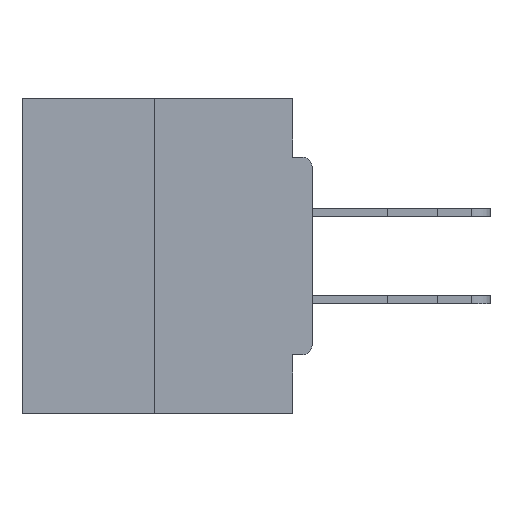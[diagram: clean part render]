
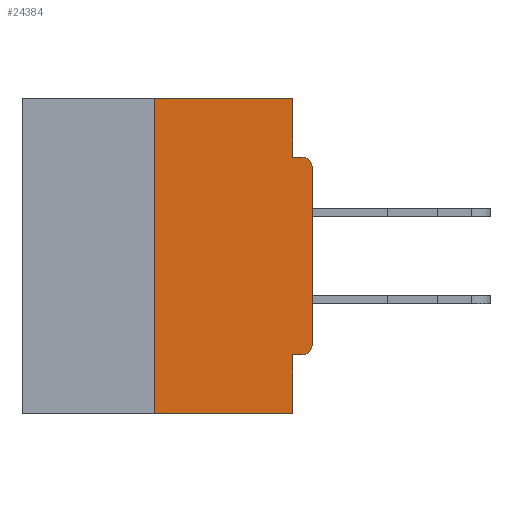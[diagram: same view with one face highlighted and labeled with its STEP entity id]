
A CAD part, left-side view. The second image highlights one B-rep face of the part: STEP entity #24384.
In plain terms, the highlighted planar face has unit normal (-1, 0, 0).
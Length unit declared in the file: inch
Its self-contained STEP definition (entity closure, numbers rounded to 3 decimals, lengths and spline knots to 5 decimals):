
#837 = DIRECTION ( 'NONE',  ( 0., 0., -1. ) ) ;
#1456 = LINE ( 'NONE', #22021, #6409 ) ;
#1911 = AXIS2_PLACEMENT_3D ( 'NONE', #15121, #15241, #32262 ) ;
#2408 = DIRECTION ( 'NONE',  ( 0., 0., -1. ) ) ;
#2849 = CARTESIAN_POINT ( 'NONE',  ( 0., 0.031, -0.4065 ) ) ;
#3542 = VECTOR ( 'NONE', #2408, 39.37008 ) ;
#3547 = VERTEX_POINT ( 'NONE', #22364 ) ;
#3574 = DIRECTION ( 'NONE',  ( -1., 0., 0. ) ) ;
#3771 = DIRECTION ( 'NONE',  ( 0., 1., 0. ) ) ;
#4537 = ORIENTED_EDGE ( 'NONE', *, *, #19357, .F. ) ;
#5970 = VERTEX_POINT ( 'NONE', #33038 ) ;
#6409 = VECTOR ( 'NONE', #3771, 39.37008 ) ;
#6450 = VECTOR ( 'NONE', #30759, 39.37008 ) ;
#7150 = DIRECTION ( 'NONE',  ( 0., 0., 1. ) ) ;
#7589 = LINE ( 'NONE', #16552, #3542 ) ;
#7725 = CARTESIAN_POINT ( 'NONE',  ( 0., 0.46, -0.5 ) ) ;
#9317 = DIRECTION ( 'NONE',  ( 0., -1., 0. ) ) ;
#9346 = EDGE_CURVE ( 'NONE', #17572, #32193, #27491, .T. ) ;
#9923 = ORIENTED_EDGE ( 'NONE', *, *, #14811, .T. ) ;
#10273 = ORIENTED_EDGE ( 'NONE', *, *, #27734, .F. ) ;
#11544 = LINE ( 'NONE', #16419, #13365 ) ;
#11644 = DIRECTION ( 'NONE',  ( 0., -1., 0. ) ) ;
#11818 = LINE ( 'NONE', #21107, #30817 ) ;
#12034 = CARTESIAN_POINT ( 'NONE',  ( 0., 0., -0.3915 ) ) ;
#12167 = AXIS2_PLACEMENT_3D ( 'NONE', #26490, #3574, #837 ) ;
#12529 = DIRECTION ( 'NONE',  ( 0., 0., -1. ) ) ;
#13314 = EDGE_CURVE ( 'NONE', #35030, #5970, #11818, .T. ) ;
#13365 = VECTOR ( 'NONE', #30950, 39.37008 ) ;
#14696 = CARTESIAN_POINT ( 'NONE',  ( 0., 0.015, -0.4065 ) ) ;
#14811 = EDGE_CURVE ( 'NONE', #3547, #5970, #28433, .T. ) ;
#15121 = CARTESIAN_POINT ( 'NONE',  ( 0., 0.015, -0.3915 ) ) ;
#15241 = DIRECTION ( 'NONE',  ( -1., 0., 0. ) ) ;
#15421 = PLANE ( 'NONE',  #22726 ) ;
#16419 = CARTESIAN_POINT ( 'NONE',  ( 0., 0., 0. ) ) ;
#16548 = LINE ( 'NONE', #17117, #25144 ) ;
#16552 = CARTESIAN_POINT ( 'NONE',  ( 0., 0.031, 0. ) ) ;
#16988 = DIRECTION ( 'NONE',  ( 0., 0., -1. ) ) ;
#17117 = CARTESIAN_POINT ( 'NONE',  ( 0., 0.031, -0.5 ) ) ;
#17572 = VERTEX_POINT ( 'NONE', #14696 ) ;
#19357 = EDGE_CURVE ( 'NONE', #35342, #22107, #31968, .T. ) ;
#19617 = VECTOR ( 'NONE', #11644, 39.37008 ) ;
#19717 = EDGE_CURVE ( 'NONE', #37078, #26133, #16548, .T. ) ;
#21019 = LINE ( 'NONE', #26024, #19617 ) ;
#21107 = CARTESIAN_POINT ( 'NONE',  ( 0., 0., -0.0935 ) ) ;
#21246 = ORIENTED_EDGE ( 'NONE', *, *, #9346, .T. ) ;
#21857 = ORIENTED_EDGE ( 'NONE', *, *, #22787, .F. ) ;
#22021 = CARTESIAN_POINT ( 'NONE',  ( 0., 0., -0.4065 ) ) ;
#22107 = VERTEX_POINT ( 'NONE', #24955 ) ;
#22237 = CARTESIAN_POINT ( 'NONE',  ( 0., 0.031, -0.5 ) ) ;
#22364 = CARTESIAN_POINT ( 'NONE',  ( 0., 0., -0.1085 ) ) ;
#22726 = AXIS2_PLACEMENT_3D ( 'NONE', #24101, #32914, #12529 ) ;
#22787 = EDGE_CURVE ( 'NONE', #17572, #37078, #1456, .T. ) ;
#23242 = ORIENTED_EDGE ( 'NONE', *, *, #13314, .F. ) ;
#24101 = CARTESIAN_POINT ( 'NONE',  ( 0., 0.46, 0. ) ) ;
#24384 = ADVANCED_FACE ( 'NONE', ( #34598 ), #15421, .F. ) ;
#24397 = CARTESIAN_POINT ( 'NONE',  ( 0., 0.031, 0. ) ) ;
#24955 = CARTESIAN_POINT ( 'NONE',  ( 0., 0.25, 0. ) ) ;
#25144 = VECTOR ( 'NONE', #16988, 39.37008 ) ;
#25373 = CARTESIAN_POINT ( 'NONE',  ( 0., 0.031, -0.0935 ) ) ;
#26024 = CARTESIAN_POINT ( 'NONE',  ( 0., 0.46, 0. ) ) ;
#26133 = VERTEX_POINT ( 'NONE', #22237 ) ;
#26490 = CARTESIAN_POINT ( 'NONE',  ( 0., 0.015, -0.1085 ) ) ;
#26702 = LINE ( 'NONE', #7725, #6450 ) ;
#27491 = CIRCLE ( 'NONE', #1911, 0.015 ) ;
#27734 = EDGE_CURVE ( 'NONE', #34871, #35030, #7589, .T. ) ;
#28433 = CIRCLE ( 'NONE', #12167, 0.015 ) ;
#29302 = EDGE_CURVE ( 'NONE', #22107, #34871, #21019, .T. ) ;
#30649 = CARTESIAN_POINT ( 'NONE',  ( 0., 0.25, -0.5 ) ) ;
#30711 = ORIENTED_EDGE ( 'NONE', *, *, #29302, .F. ) ;
#30759 = DIRECTION ( 'NONE',  ( 0., -1., 0. ) ) ;
#30817 = VECTOR ( 'NONE', #9317, 39.37008 ) ;
#30950 = DIRECTION ( 'NONE',  ( 0., 0., 1. ) ) ;
#31752 = EDGE_CURVE ( 'NONE', #35342, #26133, #26702, .T. ) ;
#31968 = LINE ( 'NONE', #36042, #35516 ) ;
#32193 = VERTEX_POINT ( 'NONE', #12034 ) ;
#32262 = DIRECTION ( 'NONE',  ( 0., 0., -1. ) ) ;
#32849 = ORIENTED_EDGE ( 'NONE', *, *, #31752, .T. ) ;
#32914 = DIRECTION ( 'NONE',  ( 1., 0., 0. ) ) ;
#33038 = CARTESIAN_POINT ( 'NONE',  ( 0., 0.015, -0.0935 ) ) ;
#34282 = ORIENTED_EDGE ( 'NONE', *, *, #34371, .T. ) ;
#34371 = EDGE_CURVE ( 'NONE', #32193, #3547, #11544, .T. ) ;
#34598 = FACE_OUTER_BOUND ( 'NONE', #35817, .T. ) ;
#34871 = VERTEX_POINT ( 'NONE', #24397 ) ;
#35030 = VERTEX_POINT ( 'NONE', #25373 ) ;
#35342 = VERTEX_POINT ( 'NONE', #30649 ) ;
#35516 = VECTOR ( 'NONE', #7150, 39.37008 ) ;
#35817 = EDGE_LOOP ( 'NONE', ( #30711, #4537, #32849, #36057, #21857, #21246, #34282, #9923, #23242, #10273 ) ) ;
#36042 = CARTESIAN_POINT ( 'NONE',  ( 0., 0.25, 0. ) ) ;
#36057 = ORIENTED_EDGE ( 'NONE', *, *, #19717, .F. ) ;
#37078 = VERTEX_POINT ( 'NONE', #2849 ) ;
